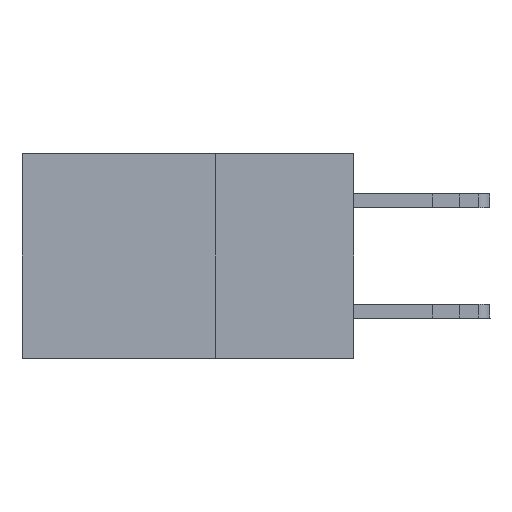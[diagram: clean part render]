
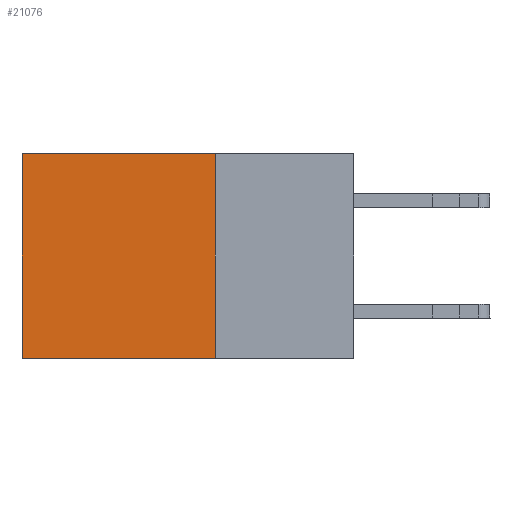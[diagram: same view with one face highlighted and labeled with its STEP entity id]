
A CAD part, left-side view. The second image highlights one B-rep face of the part: STEP entity #21076.
In plain terms, the highlighted planar face has unit normal (-1, 0, 0).
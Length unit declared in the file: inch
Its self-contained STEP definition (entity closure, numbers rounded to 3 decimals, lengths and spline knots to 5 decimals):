
#1507 = CARTESIAN_POINT ( 'NONE',  ( 0.2875, 0.25, 0. ) ) ;
#1803 = ORIENTED_EDGE ( 'NONE', *, *, #19236, .F. ) ;
#2741 = VERTEX_POINT ( 'NONE', #17485 ) ;
#5940 = CARTESIAN_POINT ( 'NONE',  ( 0.2875, 0.25, 0. ) ) ;
#6227 = LINE ( 'NONE', #12891, #20129 ) ;
#7530 = DIRECTION ( 'NONE',  ( 0., 1., 0. ) ) ;
#8666 = ORIENTED_EDGE ( 'NONE', *, *, #13425, .T. ) ;
#8768 = VECTOR ( 'NONE', #7530, 39.37008 ) ;
#8798 = EDGE_CURVE ( 'NONE', #2741, #10054, #27451, .T. ) ;
#10054 = VERTEX_POINT ( 'NONE', #28889 ) ;
#10760 = DIRECTION ( 'NONE',  ( 0., 0., -1. ) ) ;
#11784 = ORIENTED_EDGE ( 'NONE', *, *, #19662, .F. ) ;
#12360 = VECTOR ( 'NONE', #19911, 39.37008 ) ;
#12699 = LINE ( 'NONE', #16612, #8768 ) ;
#12785 = DIRECTION ( 'NONE',  ( 0., 0., -1. ) ) ;
#12891 = CARTESIAN_POINT ( 'NONE',  ( 0.2875, 0.25, 0. ) ) ;
#13050 = CARTESIAN_POINT ( 'NONE',  ( 0.2875, 0.25, 0. ) ) ;
#13425 = EDGE_CURVE ( 'NONE', #26904, #2741, #6227, .T. ) ;
#15239 = PLANE ( 'NONE',  #24904 ) ;
#15510 = FACE_OUTER_BOUND ( 'NONE', #20290, .T. ) ;
#16612 = CARTESIAN_POINT ( 'NONE',  ( 0.2875, 0.25, -0.37 ) ) ;
#17485 = CARTESIAN_POINT ( 'NONE',  ( 0.2875, 0.6, 0. ) ) ;
#18404 = ORIENTED_EDGE ( 'NONE', *, *, #8798, .T. ) ;
#19236 = EDGE_CURVE ( 'NONE', #26904, #22351, #26204, .T. ) ;
#19554 = DIRECTION ( 'NONE',  ( 0., 1., 0. ) ) ;
#19662 = EDGE_CURVE ( 'NONE', #22351, #10054, #12699, .T. ) ;
#19700 = DIRECTION ( 'NONE',  ( 1., 0., 0. ) ) ;
#19911 = DIRECTION ( 'NONE',  ( 0., 0., -1. ) ) ;
#20129 = VECTOR ( 'NONE', #19554, 39.37008 ) ;
#20290 = EDGE_LOOP ( 'NONE', ( #18404, #11784, #1803, #8666 ) ) ;
#21076 = ADVANCED_FACE ( 'NONE', ( #15510 ), #15239, .F. ) ;
#21564 = CARTESIAN_POINT ( 'NONE',  ( 0.2875, 0.25, -0.37 ) ) ;
#22351 = VERTEX_POINT ( 'NONE', #21564 ) ;
#24904 = AXIS2_PLACEMENT_3D ( 'NONE', #5940, #19700, #10760 ) ;
#25693 = VECTOR ( 'NONE', #12785, 39.37008 ) ;
#26204 = LINE ( 'NONE', #13050, #12360 ) ;
#26904 = VERTEX_POINT ( 'NONE', #1507 ) ;
#27451 = LINE ( 'NONE', #28948, #25693 ) ;
#28889 = CARTESIAN_POINT ( 'NONE',  ( 0.2875, 0.6, -0.37 ) ) ;
#28948 = CARTESIAN_POINT ( 'NONE',  ( 0.2875, 0.6, 0. ) ) ;
